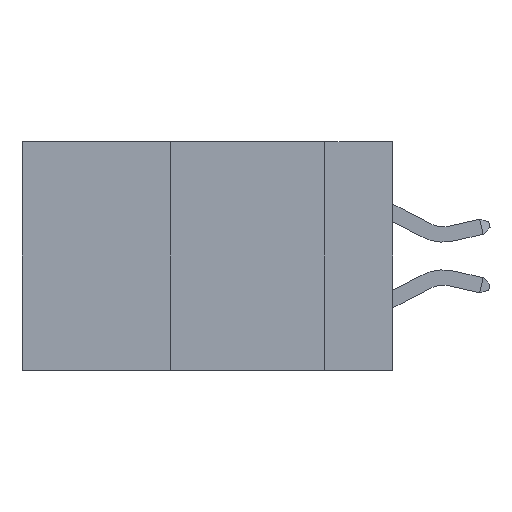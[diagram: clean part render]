
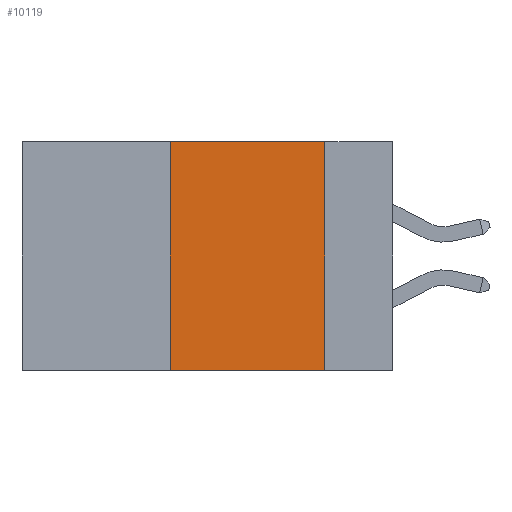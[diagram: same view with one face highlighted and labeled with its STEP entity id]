
A CAD part, left-side view. The second image highlights one B-rep face of the part: STEP entity #10119.
In plain terms, the highlighted planar face has unit normal (-1, 0, 0).
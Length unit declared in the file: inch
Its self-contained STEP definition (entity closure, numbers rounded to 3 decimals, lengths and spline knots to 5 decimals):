
#1000 = VECTOR ( 'NONE', #14068, 39.37008 ) ;
#1203 = ORIENTED_EDGE ( 'NONE', *, *, #4024, .F. ) ;
#2086 = VERTEX_POINT ( 'NONE', #13705 ) ;
#2257 = DIRECTION ( 'NONE',  ( 0., 0., -1. ) ) ;
#3964 = CARTESIAN_POINT ( 'NONE',  ( 0., 0.11, 0. ) ) ;
#3978 = DIRECTION ( 'NONE',  ( 0., 0., -1. ) ) ;
#4024 = EDGE_CURVE ( 'NONE', #4793, #15588, #12778, .T. ) ;
#4256 = VECTOR ( 'NONE', #7587, 39.37008 ) ;
#4654 = DIRECTION ( 'NONE',  ( 1., 0., 0. ) ) ;
#4681 = DIRECTION ( 'NONE',  ( 0., 0., 1. ) ) ;
#4687 = ORIENTED_EDGE ( 'NONE', *, *, #7970, .T. ) ;
#4793 = VERTEX_POINT ( 'NONE', #3964 ) ;
#5385 = CARTESIAN_POINT ( 'NONE',  ( 0., 0.36, 0. ) ) ;
#6059 = LINE ( 'NONE', #8519, #10945 ) ;
#6245 = EDGE_CURVE ( 'NONE', #12631, #4793, #15176, .T. ) ;
#6921 = CARTESIAN_POINT ( 'NONE',  ( 0., 0.6, 0. ) ) ;
#7551 = CARTESIAN_POINT ( 'NONE',  ( 0., 0.11, 0. ) ) ;
#7587 = DIRECTION ( 'NONE',  ( 0., -1., 0. ) ) ;
#7970 = EDGE_CURVE ( 'NONE', #2086, #15588, #8580, .T. ) ;
#8279 = CARTESIAN_POINT ( 'NONE',  ( 0., 0.6, 0. ) ) ;
#8402 = CARTESIAN_POINT ( 'NONE',  ( 0., 0.11, -0.37 ) ) ;
#8519 = CARTESIAN_POINT ( 'NONE',  ( 0., 0.36, 0. ) ) ;
#8580 = LINE ( 'NONE', #8805, #4256 ) ;
#8805 = CARTESIAN_POINT ( 'NONE',  ( 0., 0.6, -0.37 ) ) ;
#9640 = AXIS2_PLACEMENT_3D ( 'NONE', #8279, #4654, #2257 ) ;
#9718 = EDGE_CURVE ( 'NONE', #2086, #12631, #6059, .T. ) ;
#10119 = ADVANCED_FACE ( 'NONE', ( #12975 ), #14167, .F. ) ;
#10945 = VECTOR ( 'NONE', #4681, 39.37008 ) ;
#11531 = ORIENTED_EDGE ( 'NONE', *, *, #9718, .F. ) ;
#12063 = EDGE_LOOP ( 'NONE', ( #1203, #15288, #11531, #4687 ) ) ;
#12208 = VECTOR ( 'NONE', #3978, 39.37008 ) ;
#12631 = VERTEX_POINT ( 'NONE', #5385 ) ;
#12778 = LINE ( 'NONE', #7551, #12208 ) ;
#12975 = FACE_OUTER_BOUND ( 'NONE', #12063, .T. ) ;
#13705 = CARTESIAN_POINT ( 'NONE',  ( 0., 0.36, -0.37 ) ) ;
#14068 = DIRECTION ( 'NONE',  ( 0., -1., 0. ) ) ;
#14167 = PLANE ( 'NONE',  #9640 ) ;
#15176 = LINE ( 'NONE', #6921, #1000 ) ;
#15288 = ORIENTED_EDGE ( 'NONE', *, *, #6245, .F. ) ;
#15588 = VERTEX_POINT ( 'NONE', #8402 ) ;
